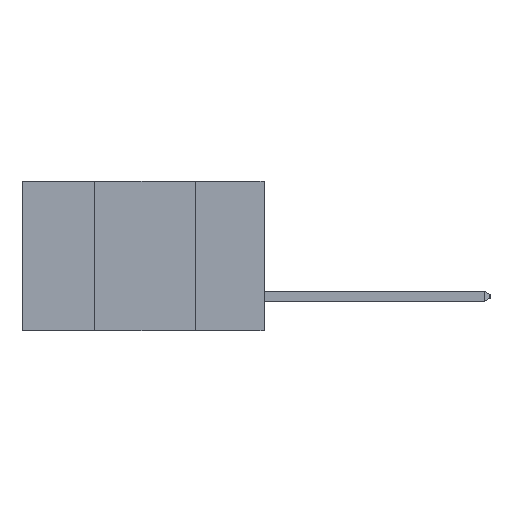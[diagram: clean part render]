
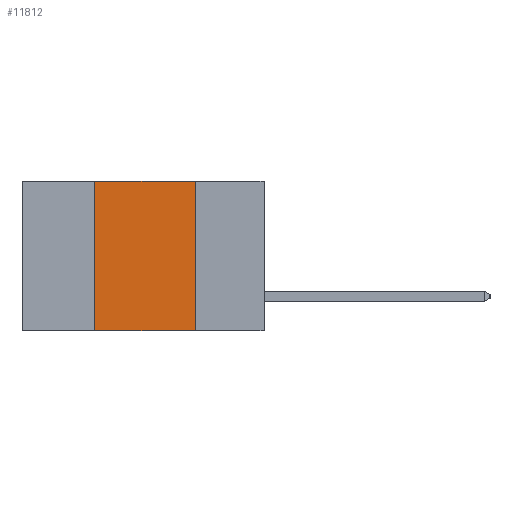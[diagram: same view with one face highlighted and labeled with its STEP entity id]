
A CAD part, left-side view. The second image highlights one B-rep face of the part: STEP entity #11812.
In plain terms, the highlighted planar face has unit normal (-1, 0, 0).
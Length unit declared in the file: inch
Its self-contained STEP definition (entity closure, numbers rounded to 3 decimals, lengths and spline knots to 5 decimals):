
#193 = PLANE ( 'NONE',  #7236 ) ;
#200 = CARTESIAN_POINT ( 'NONE',  ( 0., 0.17, -0.37 ) ) ;
#381 = LINE ( 'NONE', #1964, #10078 ) ;
#721 = EDGE_CURVE ( 'NONE', #3367, #950, #9345, .T. ) ;
#950 = VERTEX_POINT ( 'NONE', #5792 ) ;
#1183 = ORIENTED_EDGE ( 'NONE', *, *, #5930, .F. ) ;
#1195 = DIRECTION ( 'NONE',  ( 0., 0., -1. ) ) ;
#1350 = VECTOR ( 'NONE', #9373, 39.37008 ) ;
#1434 = ORIENTED_EDGE ( 'NONE', *, *, #721, .F. ) ;
#1742 = LINE ( 'NONE', #10955, #8919 ) ;
#1816 = CARTESIAN_POINT ( 'NONE',  ( 0., 0.42, -0.37 ) ) ;
#1830 = ORIENTED_EDGE ( 'NONE', *, *, #9174, .T. ) ;
#1906 = DIRECTION ( 'NONE',  ( 0., -1., 0. ) ) ;
#1914 = VECTOR ( 'NONE', #3728, 39.37008 ) ;
#1964 = CARTESIAN_POINT ( 'NONE',  ( 0., 0.6, 0. ) ) ;
#3130 = CARTESIAN_POINT ( 'NONE',  ( 0., 0.6, 0. ) ) ;
#3332 = CARTESIAN_POINT ( 'NONE',  ( 0., 0.42, -0.37 ) ) ;
#3367 = VERTEX_POINT ( 'NONE', #1816 ) ;
#3518 = VERTEX_POINT ( 'NONE', #5484 ) ;
#3728 = DIRECTION ( 'NONE',  ( 0., 0., 1. ) ) ;
#3864 = CARTESIAN_POINT ( 'NONE',  ( 0., 0.6, -0.37 ) ) ;
#4754 = EDGE_LOOP ( 'NONE', ( #7287, #1183, #1434, #1830 ) ) ;
#4794 = FACE_OUTER_BOUND ( 'NONE', #4754, .T. ) ;
#5484 = CARTESIAN_POINT ( 'NONE',  ( 0., 0.17, 0. ) ) ;
#5792 = CARTESIAN_POINT ( 'NONE',  ( 0., 0.42, 0. ) ) ;
#5930 = EDGE_CURVE ( 'NONE', #950, #3518, #381, .T. ) ;
#6167 = LINE ( 'NONE', #3864, #1350 ) ;
#6200 = VERTEX_POINT ( 'NONE', #200 ) ;
#6937 = DIRECTION ( 'NONE',  ( 1., 0., 0. ) ) ;
#7154 = EDGE_CURVE ( 'NONE', #3518, #6200, #1742, .T. ) ;
#7236 = AXIS2_PLACEMENT_3D ( 'NONE', #3130, #6937, #1195 ) ;
#7287 = ORIENTED_EDGE ( 'NONE', *, *, #7154, .F. ) ;
#8919 = VECTOR ( 'NONE', #10944, 39.37008 ) ;
#9174 = EDGE_CURVE ( 'NONE', #3367, #6200, #6167, .T. ) ;
#9345 = LINE ( 'NONE', #3332, #1914 ) ;
#9373 = DIRECTION ( 'NONE',  ( 0., -1., 0. ) ) ;
#10078 = VECTOR ( 'NONE', #1906, 39.37008 ) ;
#10944 = DIRECTION ( 'NONE',  ( 0., 0., -1. ) ) ;
#10955 = CARTESIAN_POINT ( 'NONE',  ( 0., 0.17, -0.37 ) ) ;
#11812 = ADVANCED_FACE ( 'NONE', ( #4794 ), #193, .F. ) ;
